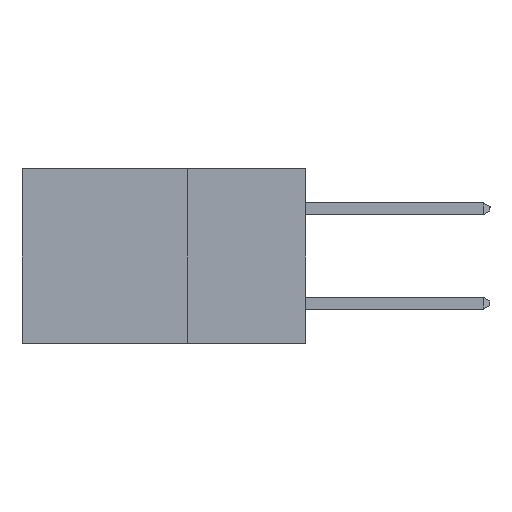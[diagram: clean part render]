
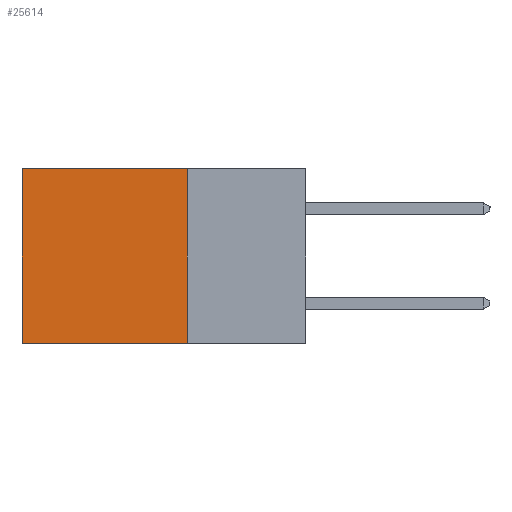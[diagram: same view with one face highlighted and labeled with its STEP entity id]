
A CAD part, left-side view. The second image highlights one B-rep face of the part: STEP entity #25614.
In plain terms, the highlighted planar face has unit normal (-1, 0, 0).
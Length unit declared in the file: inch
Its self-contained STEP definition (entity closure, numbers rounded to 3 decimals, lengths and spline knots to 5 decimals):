
#156 = VERTEX_POINT ( 'NONE', #17265 ) ;
#313 = VECTOR ( 'NONE', #5402, 39.37008 ) ;
#530 = VERTEX_POINT ( 'NONE', #2133 ) ;
#808 = LINE ( 'NONE', #3136, #13205 ) ;
#1987 = DIRECTION ( 'NONE',  ( 0., 1., 0. ) ) ;
#2133 = CARTESIAN_POINT ( 'NONE',  ( 0.2615, 0.6, 0. ) ) ;
#2500 = LINE ( 'NONE', #16025, #17852 ) ;
#2545 = DIRECTION ( 'NONE',  ( 0., 0., -1. ) ) ;
#2929 = FACE_OUTER_BOUND ( 'NONE', #6619, .T. ) ;
#3136 = CARTESIAN_POINT ( 'NONE',  ( 0.2615, 0.25, 0. ) ) ;
#3198 = EDGE_CURVE ( 'NONE', #156, #18350, #23832, .T. ) ;
#5402 = DIRECTION ( 'NONE',  ( 0., 0., -1. ) ) ;
#5888 = DIRECTION ( 'NONE',  ( 0., 0., -1. ) ) ;
#6619 = EDGE_LOOP ( 'NONE', ( #10175, #6648, #13290, #11051 ) ) ;
#6648 = ORIENTED_EDGE ( 'NONE', *, *, #22073, .F. ) ;
#8681 = AXIS2_PLACEMENT_3D ( 'NONE', #16964, #18802, #2545 ) ;
#8820 = EDGE_CURVE ( 'NONE', #530, #11729, #23211, .T. ) ;
#10175 = ORIENTED_EDGE ( 'NONE', *, *, #8820, .T. ) ;
#11051 = ORIENTED_EDGE ( 'NONE', *, *, #17987, .T. ) ;
#11729 = VERTEX_POINT ( 'NONE', #14865 ) ;
#13205 = VECTOR ( 'NONE', #21098, 39.37008 ) ;
#13290 = ORIENTED_EDGE ( 'NONE', *, *, #3198, .F. ) ;
#14865 = CARTESIAN_POINT ( 'NONE',  ( 0.2615, 0.6, -0.37 ) ) ;
#16025 = CARTESIAN_POINT ( 'NONE',  ( 0.2615, 0.25, -0.37 ) ) ;
#16963 = CARTESIAN_POINT ( 'NONE',  ( 0.2615, 0.6, -0.37 ) ) ;
#16964 = CARTESIAN_POINT ( 'NONE',  ( 0.2615, 0.25, -0.37 ) ) ;
#17265 = CARTESIAN_POINT ( 'NONE',  ( 0.2615, 0.25, 0. ) ) ;
#17852 = VECTOR ( 'NONE', #1987, 39.37008 ) ;
#17987 = EDGE_CURVE ( 'NONE', #156, #530, #808, .T. ) ;
#18350 = VERTEX_POINT ( 'NONE', #21984 ) ;
#18802 = DIRECTION ( 'NONE',  ( 1., 0., 0. ) ) ;
#20436 = VECTOR ( 'NONE', #5888, 39.37008 ) ;
#21098 = DIRECTION ( 'NONE',  ( 0., 1., 0. ) ) ;
#21984 = CARTESIAN_POINT ( 'NONE',  ( 0.2615, 0.25, -0.37 ) ) ;
#22073 = EDGE_CURVE ( 'NONE', #18350, #11729, #2500, .T. ) ;
#22564 = PLANE ( 'NONE',  #8681 ) ;
#23211 = LINE ( 'NONE', #16963, #313 ) ;
#23439 = CARTESIAN_POINT ( 'NONE',  ( 0.2615, 0.25, -0.37 ) ) ;
#23832 = LINE ( 'NONE', #23439, #20436 ) ;
#25614 = ADVANCED_FACE ( 'NONE', ( #2929 ), #22564, .F. ) ;
